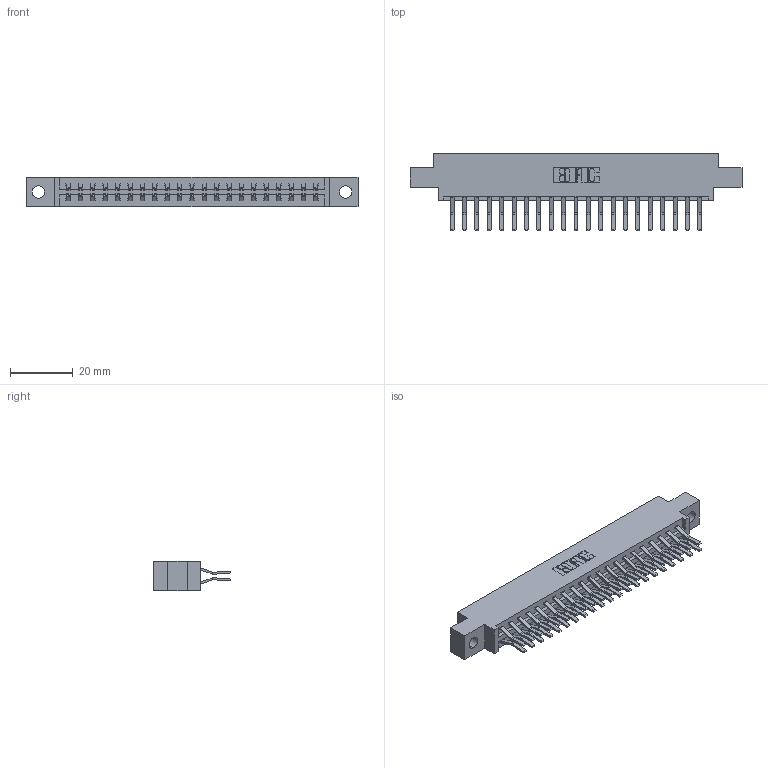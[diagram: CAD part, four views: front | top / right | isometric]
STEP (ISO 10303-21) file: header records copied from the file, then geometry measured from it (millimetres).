
FILE_DESCRIPTION (( 'STEP AP203' ), '1' );
FILE_NAME ('337-042-560-804.STEP', '2019-10-11T13:14:51', ( '' ), ( '' ), 'SwSTEP 2.0', 'SolidWorks 2016', '' );
FILE_SCHEMA (( 'CONFIG_CONTROL_DESIGN' ));
Length unit declared in the file: inch
Products named in the file (3): 345-292-001_560 Tail; 337 Part_0.170 Offset - 0.156 Dia-TH; 337-042-560-804
Assembly tree (43 placements, depth 2):
  337-042-560-804
    337 Part_0.170 Offset - 0.156 Dia-TH
    345-292-001_560 Tail  x42
Bounding box: 106.22 x 24.78 x 9.4 mm (x, y, z)
Volume: 10985 mm3; surface area: 12916.6 mm2
Topology: 43 solids, 43 shells, 2470 faces, 7337 edges, 4834 vertices
Faces by surface type: plane 1670, cylinder 800
Entity records: 19221 total; most frequent: CARTESIAN_POINT 3258, ORIENTED_EDGE 3194, DIRECTION 2813, EDGE_CURVE 1597, LINE 1465, VECTOR 1465, VERTEX_POINT 1062, AXIS2_PLACEMENT_3D 674
